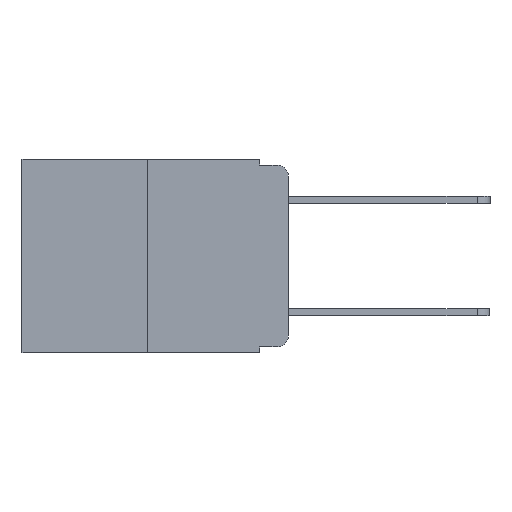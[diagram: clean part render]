
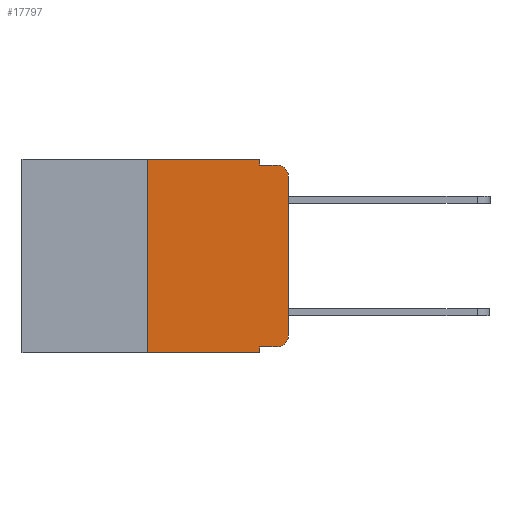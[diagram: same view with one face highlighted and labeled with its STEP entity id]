
A CAD part, left-side view. The second image highlights one B-rep face of the part: STEP entity #17797.
In plain terms, the highlighted planar face has unit normal (-1, 0, 0).
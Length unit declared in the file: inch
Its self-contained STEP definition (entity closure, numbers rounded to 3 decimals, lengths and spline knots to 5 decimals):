
#608 = CARTESIAN_POINT ( 'NONE',  ( 0., 0.051, 0. ) ) ;
#612 = DIRECTION ( 'NONE',  ( 0., -1., 0. ) ) ;
#691 = DIRECTION ( 'NONE',  ( 0., 0., -1. ) ) ;
#1033 = CARTESIAN_POINT ( 'NONE',  ( 0., 0.25, -0.343 ) ) ;
#1057 = DIRECTION ( 'NONE',  ( -1., 0., 0. ) ) ;
#1200 = ORIENTED_EDGE ( 'NONE', *, *, #19584, .F. ) ;
#1214 = DIRECTION ( 'NONE',  ( 0., -1., 0. ) ) ;
#1635 = DIRECTION ( 'NONE',  ( 1., 0., 0. ) ) ;
#2420 = LINE ( 'NONE', #19561, #10700 ) ;
#2716 = LINE ( 'NONE', #11043, #19067 ) ;
#2979 = DIRECTION ( 'NONE',  ( 0., 0., 1. ) ) ;
#3065 = AXIS2_PLACEMENT_3D ( 'NONE', #11525, #1635, #13073 ) ;
#3077 = CARTESIAN_POINT ( 'NONE',  ( 0., 0.02, -0.03 ) ) ;
#3113 = VERTEX_POINT ( 'NONE', #17010 ) ;
#3167 = VERTEX_POINT ( 'NONE', #11954 ) ;
#4248 = LINE ( 'NONE', #6441, #15966 ) ;
#4468 = VERTEX_POINT ( 'NONE', #9270 ) ;
#4822 = DIRECTION ( 'NONE',  ( 0., 0., -1. ) ) ;
#4982 = CARTESIAN_POINT ( 'NONE',  ( 0., 0.051, 0. ) ) ;
#5735 = VECTOR ( 'NONE', #612, 39.37008 ) ;
#5815 = CARTESIAN_POINT ( 'NONE',  ( 0., 0.02, -0.01 ) ) ;
#5986 = AXIS2_PLACEMENT_3D ( 'NONE', #3077, #14390, #4822 ) ;
#6222 = DIRECTION ( 'NONE',  ( 0., 0., 1. ) ) ;
#6314 = AXIS2_PLACEMENT_3D ( 'NONE', #11072, #1057, #12615 ) ;
#6441 = CARTESIAN_POINT ( 'NONE',  ( 0., 0.051, 0. ) ) ;
#6518 = EDGE_CURVE ( 'NONE', #7034, #14839, #16525, .T. ) ;
#6755 = PLANE ( 'NONE',  #3065 ) ;
#6970 = VECTOR ( 'NONE', #9483, 39.37008 ) ;
#7019 = EDGE_CURVE ( 'NONE', #4468, #7034, #2716, .T. ) ;
#7034 = VERTEX_POINT ( 'NONE', #7906 ) ;
#7247 = CARTESIAN_POINT ( 'NONE',  ( 0., 0.25, 0. ) ) ;
#7318 = ORIENTED_EDGE ( 'NONE', *, *, #14183, .T. ) ;
#7489 = ORIENTED_EDGE ( 'NONE', *, *, #7019, .T. ) ;
#7585 = EDGE_CURVE ( 'NONE', #8167, #14839, #2420, .T. ) ;
#7906 = CARTESIAN_POINT ( 'NONE',  ( 0., 0., -0.03 ) ) ;
#8167 = VERTEX_POINT ( 'NONE', #12897 ) ;
#8602 = VECTOR ( 'NONE', #691, 39.37008 ) ;
#8657 = ORIENTED_EDGE ( 'NONE', *, *, #20098, .F. ) ;
#9270 = CARTESIAN_POINT ( 'NONE',  ( 0., 0., -0.313 ) ) ;
#9370 = EDGE_CURVE ( 'NONE', #10580, #4468, #11438, .T. ) ;
#9483 = DIRECTION ( 'NONE',  ( 0., -1., 0. ) ) ;
#9786 = VERTEX_POINT ( 'NONE', #7247 ) ;
#9862 = ORIENTED_EDGE ( 'NONE', *, *, #7585, .F. ) ;
#9907 = ORIENTED_EDGE ( 'NONE', *, *, #15595, .F. ) ;
#10063 = VECTOR ( 'NONE', #1214, 39.37008 ) ;
#10411 = ORIENTED_EDGE ( 'NONE', *, *, #17682, .F. ) ;
#10580 = VERTEX_POINT ( 'NONE', #18116 ) ;
#10700 = VECTOR ( 'NONE', #20208, 39.37008 ) ;
#10738 = CARTESIAN_POINT ( 'NONE',  ( 0., 0.473, -0.343 ) ) ;
#10972 = VERTEX_POINT ( 'NONE', #4982 ) ;
#11043 = CARTESIAN_POINT ( 'NONE',  ( 0., 0., 0. ) ) ;
#11072 = CARTESIAN_POINT ( 'NONE',  ( 0., 0.02, -0.313 ) ) ;
#11438 = CIRCLE ( 'NONE', #6314, 0.02 ) ;
#11525 = CARTESIAN_POINT ( 'NONE',  ( 0., 0.473, 0. ) ) ;
#11954 = CARTESIAN_POINT ( 'NONE',  ( 0., 0.051, -0.343 ) ) ;
#12615 = DIRECTION ( 'NONE',  ( 0., 0., -1. ) ) ;
#12745 = LINE ( 'NONE', #608, #8602 ) ;
#12897 = CARTESIAN_POINT ( 'NONE',  ( 0., 0.051, -0.01 ) ) ;
#13073 = DIRECTION ( 'NONE',  ( 0., 0., -1. ) ) ;
#13309 = VECTOR ( 'NONE', #2979, 39.37008 ) ;
#13891 = FACE_OUTER_BOUND ( 'NONE', #14523, .T. ) ;
#14183 = EDGE_CURVE ( 'NONE', #14383, #3167, #14658, .T. ) ;
#14383 = VERTEX_POINT ( 'NONE', #1033 ) ;
#14390 = DIRECTION ( 'NONE',  ( -1., 0., 0. ) ) ;
#14523 = EDGE_LOOP ( 'NONE', ( #7489, #20280, #9862, #9907, #10411, #1200, #7318, #8657, #20300, #17542 ) ) ;
#14658 = LINE ( 'NONE', #10738, #5735 ) ;
#14834 = LINE ( 'NONE', #18709, #6970 ) ;
#14839 = VERTEX_POINT ( 'NONE', #5815 ) ;
#15595 = EDGE_CURVE ( 'NONE', #10972, #8167, #12745, .T. ) ;
#15966 = VECTOR ( 'NONE', #18833, 39.37008 ) ;
#16298 = LINE ( 'NONE', #17411, #10063 ) ;
#16525 = CIRCLE ( 'NONE', #5986, 0.02 ) ;
#17010 = CARTESIAN_POINT ( 'NONE',  ( 0., 0.051, -0.333 ) ) ;
#17369 = LINE ( 'NONE', #18781, #13309 ) ;
#17411 = CARTESIAN_POINT ( 'NONE',  ( 0., 0.473, 0. ) ) ;
#17542 = ORIENTED_EDGE ( 'NONE', *, *, #9370, .T. ) ;
#17682 = EDGE_CURVE ( 'NONE', #9786, #10972, #16298, .T. ) ;
#17797 = ADVANCED_FACE ( 'NONE', ( #13891 ), #6755, .F. ) ;
#18116 = CARTESIAN_POINT ( 'NONE',  ( 0., 0.02, -0.333 ) ) ;
#18599 = EDGE_CURVE ( 'NONE', #3113, #10580, #14834, .T. ) ;
#18709 = CARTESIAN_POINT ( 'NONE',  ( 0., 0.051, -0.333 ) ) ;
#18781 = CARTESIAN_POINT ( 'NONE',  ( 0., 0.25, 0. ) ) ;
#18833 = DIRECTION ( 'NONE',  ( 0., 0., -1. ) ) ;
#19067 = VECTOR ( 'NONE', #6222, 39.37008 ) ;
#19561 = CARTESIAN_POINT ( 'NONE',  ( 0., 0.051, -0.01 ) ) ;
#19584 = EDGE_CURVE ( 'NONE', #14383, #9786, #17369, .T. ) ;
#20098 = EDGE_CURVE ( 'NONE', #3113, #3167, #4248, .T. ) ;
#20208 = DIRECTION ( 'NONE',  ( 0., -1., 0. ) ) ;
#20280 = ORIENTED_EDGE ( 'NONE', *, *, #6518, .T. ) ;
#20300 = ORIENTED_EDGE ( 'NONE', *, *, #18599, .T. ) ;
